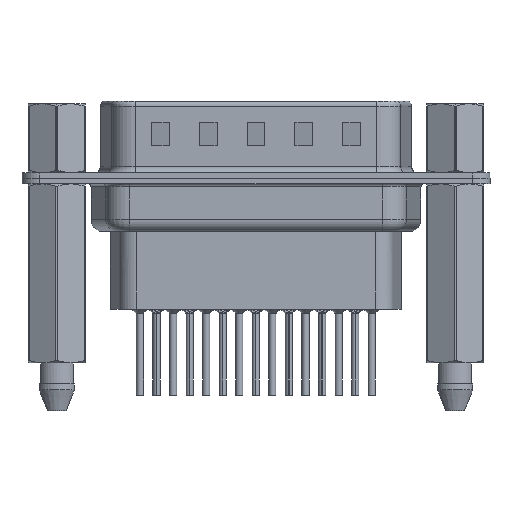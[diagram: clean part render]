
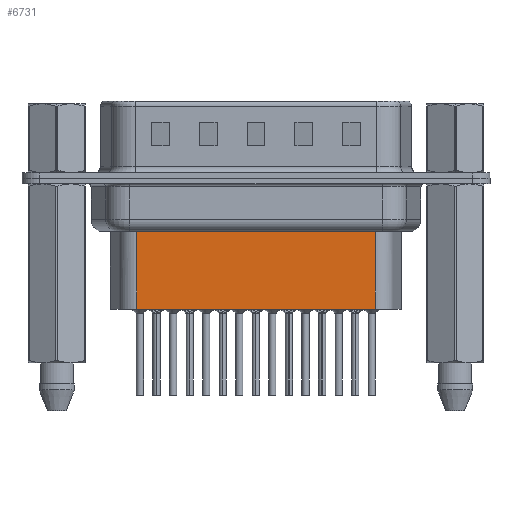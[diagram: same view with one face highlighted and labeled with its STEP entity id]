
A CAD part, front view. The second image highlights one B-rep face of the part: STEP entity #6731.
In plain terms, the highlighted planar face has unit normal (0, -1, 0).
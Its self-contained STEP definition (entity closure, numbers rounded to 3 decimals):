
#589 = EDGE_CURVE ( 'NONE', #7489, #6150, #15405, .T. ) ;
#1385 = LINE ( 'NONE', #28343, #15281 ) ;
#1425 = ORIENTED_EDGE ( 'NONE', *, *, #589, .F. ) ;
#2341 = CARTESIAN_POINT ( 'NONE',  ( 26.619, -3.5, -4.097 ) ) ;
#6049 = PLANE ( 'NONE',  #26904 ) ;
#6150 = VERTEX_POINT ( 'NONE', #20783 ) ;
#6372 = DIRECTION ( 'NONE',  ( 0., 0., -1. ) ) ;
#6677 = EDGE_CURVE ( 'NONE', #7489, #8469, #1385, .T. ) ;
#6731 = ADVANCED_FACE ( 'NONE', ( #10138 ), #6049, .T. ) ;
#7255 = CARTESIAN_POINT ( 'NONE',  ( 6.681, -3.5, -3.1 ) ) ;
#7489 = VERTEX_POINT ( 'NONE', #2341 ) ;
#7531 = LINE ( 'NONE', #7255, #19776 ) ;
#8098 = CARTESIAN_POINT ( 'NONE',  ( 6.681, -3.5, -3.1 ) ) ;
#8469 = VERTEX_POINT ( 'NONE', #20345 ) ;
#8610 = DIRECTION ( 'NONE',  ( -1., 0., 0. ) ) ;
#9989 = DIRECTION ( 'NONE',  ( -1., 0., 0. ) ) ;
#10132 = VERTEX_POINT ( 'NONE', #17285 ) ;
#10138 = FACE_OUTER_BOUND ( 'NONE', #26375, .T. ) ;
#12162 = ORIENTED_EDGE ( 'NONE', *, *, #6677, .T. ) ;
#12781 = DIRECTION ( 'NONE',  ( 1., 0., 0. ) ) ;
#14525 = DIRECTION ( 'NONE',  ( 0., -1., 0. ) ) ;
#15281 = VECTOR ( 'NONE', #9989, 1000. ) ;
#15405 = LINE ( 'NONE', #17863, #23604 ) ;
#16134 = DIRECTION ( 'NONE',  ( 0., 0., -1. ) ) ;
#16987 = EDGE_CURVE ( 'NONE', #8469, #10132, #7531, .T. ) ;
#17285 = CARTESIAN_POINT ( 'NONE',  ( 6.681, -3.5, -10.95 ) ) ;
#17621 = CARTESIAN_POINT ( 'NONE',  ( 6.681, -3.5, -10.95 ) ) ;
#17863 = CARTESIAN_POINT ( 'NONE',  ( 26.619, -3.5, -3.1 ) ) ;
#19658 = LINE ( 'NONE', #17621, #21327 ) ;
#19776 = VECTOR ( 'NONE', #16134, 1000. ) ;
#20345 = CARTESIAN_POINT ( 'NONE',  ( 6.681, -3.5, -4.097 ) ) ;
#20783 = CARTESIAN_POINT ( 'NONE',  ( 26.619, -3.5, -10.95 ) ) ;
#21123 = ORIENTED_EDGE ( 'NONE', *, *, #16987, .T. ) ;
#21327 = VECTOR ( 'NONE', #8610, 1000. ) ;
#23604 = VECTOR ( 'NONE', #6372, 1000. ) ;
#25782 = EDGE_CURVE ( 'NONE', #6150, #10132, #19658, .T. ) ;
#26000 = ORIENTED_EDGE ( 'NONE', *, *, #25782, .F. ) ;
#26375 = EDGE_LOOP ( 'NONE', ( #1425, #12162, #21123, #26000 ) ) ;
#26904 = AXIS2_PLACEMENT_3D ( 'NONE', #8098, #14525, #12781 ) ;
#28343 = CARTESIAN_POINT ( 'NONE',  ( 6.434, -3.5, -4.097 ) ) ;
